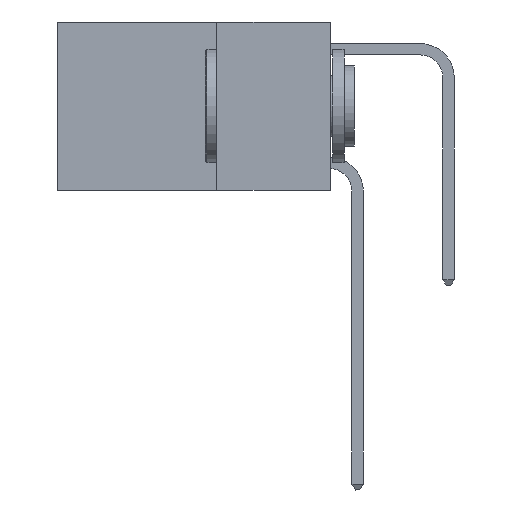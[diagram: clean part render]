
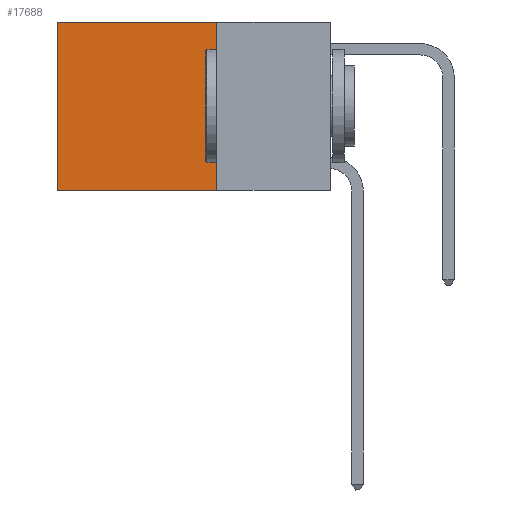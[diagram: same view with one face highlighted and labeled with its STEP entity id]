
A CAD part, left-side view. The second image highlights one B-rep face of the part: STEP entity #17688.
In plain terms, the highlighted planar face has unit normal (-1, 0, 0).
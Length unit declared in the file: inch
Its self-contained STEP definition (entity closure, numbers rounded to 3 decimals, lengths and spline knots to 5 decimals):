
#678 = EDGE_CURVE ( 'NONE', #17867, #1604, #14966, .T. ) ;
#1604 = VERTEX_POINT ( 'NONE', #11540 ) ;
#2854 = ORIENTED_EDGE ( 'NONE', *, *, #2892, .T. ) ;
#2866 = CARTESIAN_POINT ( 'NONE',  ( 0.2625, 0.25, -0.37 ) ) ;
#2892 = EDGE_CURVE ( 'NONE', #9174, #6605, #12379, .T. ) ;
#3152 = EDGE_CURVE ( 'NONE', #1604, #6605, #12328, .T. ) ;
#5758 = CARTESIAN_POINT ( 'NONE',  ( 0.2625, 0.25, 0. ) ) ;
#6605 = VERTEX_POINT ( 'NONE', #15337 ) ;
#6738 = VECTOR ( 'NONE', #8266, 39.37008 ) ;
#7111 = CARTESIAN_POINT ( 'NONE',  ( 0.2625, 0.6, 0. ) ) ;
#7237 = DIRECTION ( 'NONE',  ( 0., 0., -1. ) ) ;
#8236 = DIRECTION ( 'NONE',  ( 0., 1., 0. ) ) ;
#8266 = DIRECTION ( 'NONE',  ( 0., 1., 0. ) ) ;
#8844 = VECTOR ( 'NONE', #17039, 39.37008 ) ;
#9174 = VERTEX_POINT ( 'NONE', #7111 ) ;
#9479 = ORIENTED_EDGE ( 'NONE', *, *, #12668, .T. ) ;
#9702 = VECTOR ( 'NONE', #18082, 39.37008 ) ;
#10215 = CARTESIAN_POINT ( 'NONE',  ( 0.2625, 0.25, 0. ) ) ;
#10743 = FACE_OUTER_BOUND ( 'NONE', #18402, .T. ) ;
#11540 = CARTESIAN_POINT ( 'NONE',  ( 0.2625, 0.25, -0.37 ) ) ;
#12328 = LINE ( 'NONE', #2866, #23688 ) ;
#12379 = LINE ( 'NONE', #19786, #9702 ) ;
#12668 = EDGE_CURVE ( 'NONE', #17867, #9174, #21494, .T. ) ;
#14374 = DIRECTION ( 'NONE',  ( 1., 0., 0. ) ) ;
#14966 = LINE ( 'NONE', #5758, #8844 ) ;
#15337 = CARTESIAN_POINT ( 'NONE',  ( 0.2625, 0.6, -0.37 ) ) ;
#15742 = CARTESIAN_POINT ( 'NONE',  ( 0.2625, 0.25, 0. ) ) ;
#17039 = DIRECTION ( 'NONE',  ( 0., 0., -1. ) ) ;
#17688 = ADVANCED_FACE ( 'NONE', ( #10743 ), #18258, .F. ) ;
#17867 = VERTEX_POINT ( 'NONE', #10215 ) ;
#18082 = DIRECTION ( 'NONE',  ( 0., 0., -1. ) ) ;
#18135 = CARTESIAN_POINT ( 'NONE',  ( 0.2625, 0.25, 0. ) ) ;
#18258 = PLANE ( 'NONE',  #23306 ) ;
#18402 = EDGE_LOOP ( 'NONE', ( #2854, #18661, #21097, #9479 ) ) ;
#18661 = ORIENTED_EDGE ( 'NONE', *, *, #3152, .F. ) ;
#19786 = CARTESIAN_POINT ( 'NONE',  ( 0.2625, 0.6, 0. ) ) ;
#21097 = ORIENTED_EDGE ( 'NONE', *, *, #678, .F. ) ;
#21494 = LINE ( 'NONE', #15742, #6738 ) ;
#23306 = AXIS2_PLACEMENT_3D ( 'NONE', #18135, #14374, #7237 ) ;
#23688 = VECTOR ( 'NONE', #8236, 39.37008 ) ;
